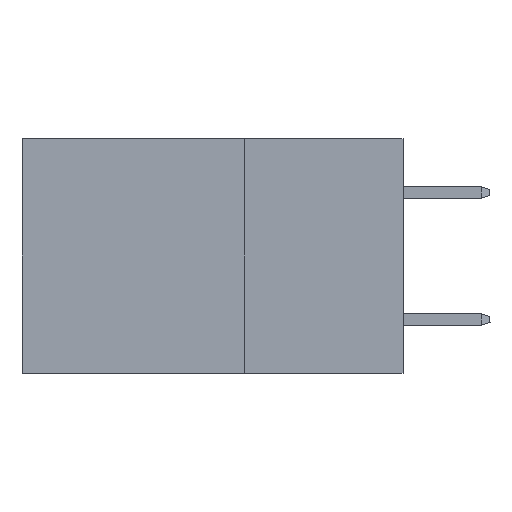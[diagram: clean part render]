
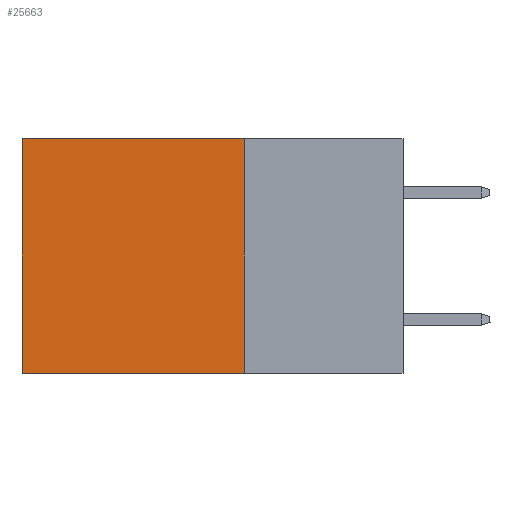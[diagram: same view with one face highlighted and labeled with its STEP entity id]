
A CAD part, left-side view. The second image highlights one B-rep face of the part: STEP entity #25663.
In plain terms, the highlighted planar face has unit normal (-1, 0, 0).
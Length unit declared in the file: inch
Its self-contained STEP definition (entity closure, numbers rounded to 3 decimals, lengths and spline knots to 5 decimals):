
#612 = DIRECTION ( 'NONE',  ( 1., 0., 0. ) ) ;
#706 = VECTOR ( 'NONE', #17649, 39.37008 ) ;
#1369 = VERTEX_POINT ( 'NONE', #25389 ) ;
#2683 = CARTESIAN_POINT ( 'NONE',  ( 0.2875, 0.25, -0.37 ) ) ;
#2929 = CARTESIAN_POINT ( 'NONE',  ( 0.2875, 0.25, 0. ) ) ;
#4188 = EDGE_CURVE ( 'NONE', #12332, #11841, #10872, .T. ) ;
#6743 = DIRECTION ( 'NONE',  ( 0., 0., -1. ) ) ;
#8840 = CARTESIAN_POINT ( 'NONE',  ( 0.2875, 0.25, 0. ) ) ;
#9769 = DIRECTION ( 'NONE',  ( 0., 1., 0. ) ) ;
#10872 = LINE ( 'NONE', #12820, #16154 ) ;
#11536 = EDGE_CURVE ( 'NONE', #12332, #13263, #11843, .T. ) ;
#11841 = VERTEX_POINT ( 'NONE', #2683 ) ;
#11843 = LINE ( 'NONE', #21369, #14251 ) ;
#12332 = VERTEX_POINT ( 'NONE', #2929 ) ;
#12820 = CARTESIAN_POINT ( 'NONE',  ( 0.2875, 0.25, 0. ) ) ;
#13263 = VERTEX_POINT ( 'NONE', #25129 ) ;
#14251 = VECTOR ( 'NONE', #9769, 39.37008 ) ;
#14453 = PLANE ( 'NONE',  #20403 ) ;
#15045 = DIRECTION ( 'NONE',  ( 0., 0., -1. ) ) ;
#15325 = EDGE_CURVE ( 'NONE', #13263, #1369, #20635, .T. ) ;
#16154 = VECTOR ( 'NONE', #15045, 39.37008 ) ;
#16219 = CARTESIAN_POINT ( 'NONE',  ( 0.2875, 0.6, 0. ) ) ;
#16479 = DIRECTION ( 'NONE',  ( 0., 0., -1. ) ) ;
#17649 = DIRECTION ( 'NONE',  ( 0., 1., 0. ) ) ;
#17651 = ORIENTED_EDGE ( 'NONE', *, *, #15325, .T. ) ;
#17783 = LINE ( 'NONE', #17908, #706 ) ;
#17908 = CARTESIAN_POINT ( 'NONE',  ( 0.2875, 0.25, -0.37 ) ) ;
#18488 = FACE_OUTER_BOUND ( 'NONE', #19601, .T. ) ;
#18620 = EDGE_CURVE ( 'NONE', #11841, #1369, #17783, .T. ) ;
#18986 = ORIENTED_EDGE ( 'NONE', *, *, #4188, .F. ) ;
#19418 = VECTOR ( 'NONE', #16479, 39.37008 ) ;
#19601 = EDGE_LOOP ( 'NONE', ( #17651, #23856, #18986, #22220 ) ) ;
#20403 = AXIS2_PLACEMENT_3D ( 'NONE', #8840, #612, #6743 ) ;
#20635 = LINE ( 'NONE', #16219, #19418 ) ;
#21369 = CARTESIAN_POINT ( 'NONE',  ( 0.2875, 0.25, 0. ) ) ;
#22220 = ORIENTED_EDGE ( 'NONE', *, *, #11536, .T. ) ;
#23856 = ORIENTED_EDGE ( 'NONE', *, *, #18620, .F. ) ;
#25129 = CARTESIAN_POINT ( 'NONE',  ( 0.2875, 0.6, 0. ) ) ;
#25389 = CARTESIAN_POINT ( 'NONE',  ( 0.2875, 0.6, -0.37 ) ) ;
#25663 = ADVANCED_FACE ( 'NONE', ( #18488 ), #14453, .F. ) ;
